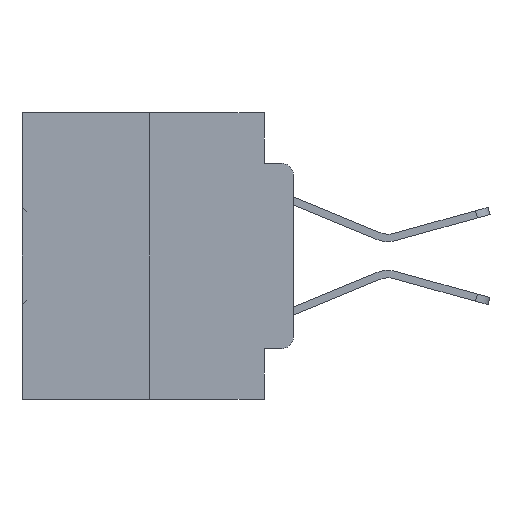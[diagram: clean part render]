
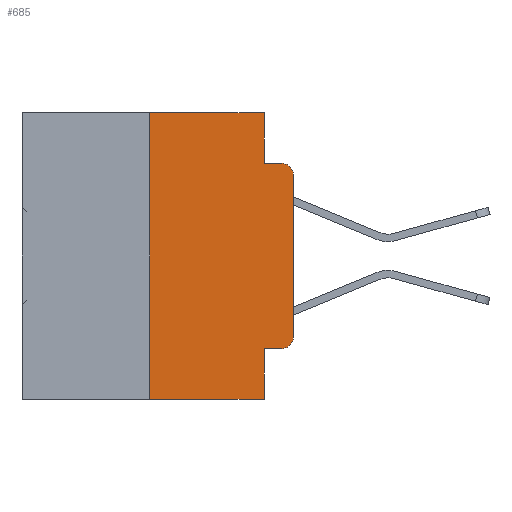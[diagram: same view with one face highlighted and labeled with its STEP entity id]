
A CAD part, left-side view. The second image highlights one B-rep face of the part: STEP entity #685.
In plain terms, the highlighted planar face has unit normal (-1, 0, 0).
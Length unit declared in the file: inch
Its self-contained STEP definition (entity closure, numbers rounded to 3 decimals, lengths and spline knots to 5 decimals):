
#685 = ADVANCED_FACE ( 'NONE', ( #32237 ), #27969, .F. ) ;
#1144 = CARTESIAN_POINT ( 'NONE',  ( 0., 0.051, 0. ) ) ;
#1591 = CARTESIAN_POINT ( 'NONE',  ( 0., 0.02, -0.4115 ) ) ;
#1645 = EDGE_CURVE ( 'NONE', #33907, #21178, #32169, .T. ) ;
#2271 = ORIENTED_EDGE ( 'NONE', *, *, #13703, .T. ) ;
#2653 = ORIENTED_EDGE ( 'NONE', *, *, #17149, .F. ) ;
#2965 = VERTEX_POINT ( 'NONE', #6381 ) ;
#3351 = CARTESIAN_POINT ( 'NONE',  ( 0., 0.051, 0. ) ) ;
#3435 = EDGE_CURVE ( 'NONE', #8791, #2965, #30136, .T. ) ;
#3548 = LINE ( 'NONE', #1144, #16868 ) ;
#3946 = ORIENTED_EDGE ( 'NONE', *, *, #26961, .T. ) ;
#4226 = LINE ( 'NONE', #24742, #17501 ) ;
#4300 = ORIENTED_EDGE ( 'NONE', *, *, #13454, .F. ) ;
#5960 = VERTEX_POINT ( 'NONE', #8350 ) ;
#6381 = CARTESIAN_POINT ( 'NONE',  ( 0., 0.02, -0.0885 ) ) ;
#7759 = DIRECTION ( 'NONE',  ( -1., 0., 0. ) ) ;
#8350 = CARTESIAN_POINT ( 'NONE',  ( 0., 0.051, -0.5 ) ) ;
#8791 = VERTEX_POINT ( 'NONE', #23330 ) ;
#8912 = ORIENTED_EDGE ( 'NONE', *, *, #18806, .T. ) ;
#9291 = CARTESIAN_POINT ( 'NONE',  ( 0., 0.473, 0. ) ) ;
#9694 = ORIENTED_EDGE ( 'NONE', *, *, #19819, .T. ) ;
#10965 = AXIS2_PLACEMENT_3D ( 'NONE', #9291, #18621, #13903 ) ;
#11303 = CARTESIAN_POINT ( 'NONE',  ( 0., 0.051, 0. ) ) ;
#11320 = AXIS2_PLACEMENT_3D ( 'NONE', #15218, #33307, #17846 ) ;
#11599 = LINE ( 'NONE', #13054, #16169 ) ;
#12629 = ORIENTED_EDGE ( 'NONE', *, *, #21364, .T. ) ;
#12775 = DIRECTION ( 'NONE',  ( 0., -1., 0. ) ) ;
#13054 = CARTESIAN_POINT ( 'NONE',  ( 0., 0.473, 0. ) ) ;
#13454 = EDGE_CURVE ( 'NONE', #19718, #8791, #3548, .T. ) ;
#13703 = EDGE_CURVE ( 'NONE', #28322, #19922, #17237, .T. ) ;
#13903 = DIRECTION ( 'NONE',  ( 0., 0., -1. ) ) ;
#13976 = DIRECTION ( 'NONE',  ( 0., 0., -1. ) ) ;
#15218 = CARTESIAN_POINT ( 'NONE',  ( 0., 0.02, -0.3915 ) ) ;
#15777 = DIRECTION ( 'NONE',  ( 0., -1., 0. ) ) ;
#16169 = VECTOR ( 'NONE', #33817, 39.37008 ) ;
#16433 = VECTOR ( 'NONE', #15777, 39.37008 ) ;
#16868 = VECTOR ( 'NONE', #17085, 39.37008 ) ;
#16903 = VECTOR ( 'NONE', #12775, 39.37008 ) ;
#17085 = DIRECTION ( 'NONE',  ( 0., 0., -1. ) ) ;
#17149 = EDGE_CURVE ( 'NONE', #28322, #5960, #32596, .T. ) ;
#17237 = LINE ( 'NONE', #30944, #16903 ) ;
#17501 = VECTOR ( 'NONE', #19650, 39.37008 ) ;
#17846 = DIRECTION ( 'NONE',  ( 0., 0., -1. ) ) ;
#18379 = CARTESIAN_POINT ( 'NONE',  ( 0., 0.051, -0.0885 ) ) ;
#18621 = DIRECTION ( 'NONE',  ( 1., 0., 0. ) ) ;
#18806 = EDGE_CURVE ( 'NONE', #30744, #2965, #28450, .T. ) ;
#19650 = DIRECTION ( 'NONE',  ( 0., 0., 1. ) ) ;
#19718 = VERTEX_POINT ( 'NONE', #3351 ) ;
#19819 = EDGE_CURVE ( 'NONE', #29300, #30744, #4226, .T. ) ;
#19922 = VERTEX_POINT ( 'NONE', #1591 ) ;
#20688 = DIRECTION ( 'NONE',  ( 0., -1., 0. ) ) ;
#21178 = VERTEX_POINT ( 'NONE', #22506 ) ;
#21364 = EDGE_CURVE ( 'NONE', #33907, #5960, #22951, .T. ) ;
#22142 = VECTOR ( 'NONE', #20688, 39.37008 ) ;
#22506 = CARTESIAN_POINT ( 'NONE',  ( 0., 0.25, 0. ) ) ;
#22676 = AXIS2_PLACEMENT_3D ( 'NONE', #23447, #7759, #26028 ) ;
#22809 = CARTESIAN_POINT ( 'NONE',  ( 0., 0.25, -0.5 ) ) ;
#22951 = LINE ( 'NONE', #25756, #22142 ) ;
#23330 = CARTESIAN_POINT ( 'NONE',  ( 0., 0.051, -0.0885 ) ) ;
#23447 = CARTESIAN_POINT ( 'NONE',  ( 0., 0.02, -0.1085 ) ) ;
#23685 = CARTESIAN_POINT ( 'NONE',  ( 0., 0., -0.3915 ) ) ;
#24046 = ORIENTED_EDGE ( 'NONE', *, *, #32796, .F. ) ;
#24316 = CARTESIAN_POINT ( 'NONE',  ( 0., 0.051, -0.4115 ) ) ;
#24742 = CARTESIAN_POINT ( 'NONE',  ( 0., 0., 0. ) ) ;
#24909 = VECTOR ( 'NONE', #13976, 39.37008 ) ;
#25212 = EDGE_LOOP ( 'NONE', ( #9694, #8912, #29656, #4300, #24046, #32555, #12629, #2653, #2271, #3946 ) ) ;
#25756 = CARTESIAN_POINT ( 'NONE',  ( 0., 0.473, -0.5 ) ) ;
#26028 = DIRECTION ( 'NONE',  ( 0., 0., -1. ) ) ;
#26220 = CIRCLE ( 'NONE', #11320, 0.02 ) ;
#26883 = VECTOR ( 'NONE', #32548, 39.37008 ) ;
#26961 = EDGE_CURVE ( 'NONE', #19922, #29300, #26220, .T. ) ;
#27969 = PLANE ( 'NONE',  #10965 ) ;
#28322 = VERTEX_POINT ( 'NONE', #24316 ) ;
#28450 = CIRCLE ( 'NONE', #22676, 0.02 ) ;
#29300 = VERTEX_POINT ( 'NONE', #23685 ) ;
#29656 = ORIENTED_EDGE ( 'NONE', *, *, #3435, .F. ) ;
#30136 = LINE ( 'NONE', #18379, #16433 ) ;
#30195 = CARTESIAN_POINT ( 'NONE',  ( 0., 0., -0.1085 ) ) ;
#30744 = VERTEX_POINT ( 'NONE', #30195 ) ;
#30944 = CARTESIAN_POINT ( 'NONE',  ( 0., 0.051, -0.4115 ) ) ;
#32169 = LINE ( 'NONE', #33803, #26883 ) ;
#32237 = FACE_OUTER_BOUND ( 'NONE', #25212, .T. ) ;
#32548 = DIRECTION ( 'NONE',  ( 0., 0., 1. ) ) ;
#32555 = ORIENTED_EDGE ( 'NONE', *, *, #1645, .F. ) ;
#32596 = LINE ( 'NONE', #11303, #24909 ) ;
#32796 = EDGE_CURVE ( 'NONE', #21178, #19718, #11599, .T. ) ;
#33307 = DIRECTION ( 'NONE',  ( -1., 0., 0. ) ) ;
#33803 = CARTESIAN_POINT ( 'NONE',  ( 0., 0.25, 0. ) ) ;
#33817 = DIRECTION ( 'NONE',  ( 0., -1., 0. ) ) ;
#33907 = VERTEX_POINT ( 'NONE', #22809 ) ;
